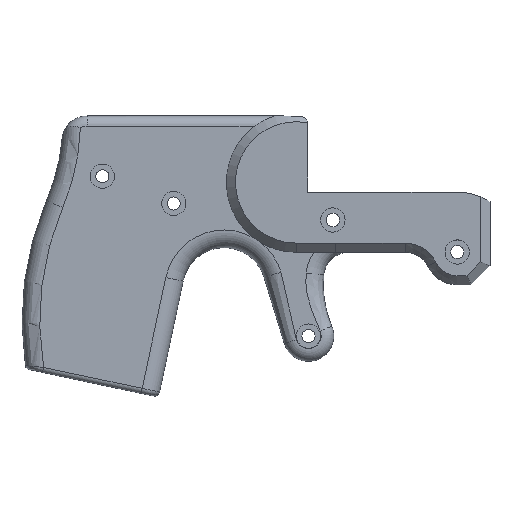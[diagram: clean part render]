
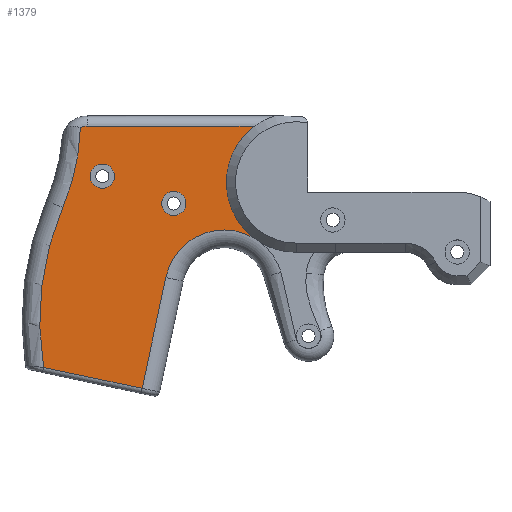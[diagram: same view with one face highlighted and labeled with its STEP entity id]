
A CAD part, top view. The second image highlights one B-rep face of the part: STEP entity #1379.
In plain terms, the highlighted planar face has unit normal (0, 0, 1).
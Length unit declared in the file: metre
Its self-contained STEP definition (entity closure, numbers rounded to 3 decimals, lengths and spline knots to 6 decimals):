
#89=LINE('',#2072,#190);
#90=LINE('',#2074,#191);
#91=LINE('',#2080,#192);
#190=VECTOR('',#1650,1.);
#191=VECTOR('',#1651,1.);
#192=VECTOR('',#1656,1.);
#291=ORIENTED_EDGE('',*,*,#693,.F.);
#292=ORIENTED_EDGE('',*,*,#694,.F.);
#293=ORIENTED_EDGE('',*,*,#695,.T.);
#294=ORIENTED_EDGE('',*,*,#696,.T.);
#295=ORIENTED_EDGE('',*,*,#697,.T.);
#296=ORIENTED_EDGE('',*,*,#698,.T.);
#297=ORIENTED_EDGE('',*,*,#699,.F.);
#298=ORIENTED_EDGE('',*,*,#700,.T.);
#299=ORIENTED_EDGE('',*,*,#701,.T.);
#300=ORIENTED_EDGE('',*,*,#702,.T.);
#693=EDGE_CURVE('',#894,#894,#1030,.T.);
#694=EDGE_CURVE('',#895,#895,#1031,.T.);
#695=EDGE_CURVE('',#896,#897,#1032,.T.);
#696=EDGE_CURVE('',#897,#898,#89,.T.);
#697=EDGE_CURVE('',#898,#899,#90,.T.);
#698=EDGE_CURVE('',#899,#900,#1033,.F.);
#699=EDGE_CURVE('',#901,#900,#1034,.T.);
#700=EDGE_CURVE('',#901,#902,#91,.F.);
#701=EDGE_CURVE('',#902,#903,#1035,.T.);
#702=EDGE_CURVE('',#903,#896,#1036,.F.);
#894=VERTEX_POINT('',#2066);
#895=VERTEX_POINT('',#2068);
#896=VERTEX_POINT('',#2070);
#897=VERTEX_POINT('',#2071);
#898=VERTEX_POINT('',#2073);
#899=VERTEX_POINT('',#2075);
#900=VERTEX_POINT('',#2077);
#901=VERTEX_POINT('',#2079);
#902=VERTEX_POINT('',#2081);
#903=VERTEX_POINT('',#2083);
#1030=CIRCLE('',#1481,0.003048);
#1031=CIRCLE('',#1482,0.003048);
#1032=CIRCLE('',#1483,0.071755);
#1033=CIRCLE('',#1484,0.014949);
#1034=CIRCLE('',#1485,0.017526);
#1035=CIRCLE('',#1486,0.00381);
#1036=CIRCLE('',#1487,0.055245);
#1101=EDGE_LOOP('',(#291));
#1102=EDGE_LOOP('',(#292));
#1103=EDGE_LOOP('',(#293,#294,#295,#296,#297,#298,#299,#300));
#1220=FACE_BOUND('',#1101,.T.);
#1221=FACE_BOUND('',#1102,.T.);
#1222=FACE_BOUND('',#1103,.T.);
#1339=PLANE('',#1480);
#1379=ADVANCED_FACE('',(#1220,#1221,#1222),#1339,.T.);
#1480=AXIS2_PLACEMENT_3D('',#2064,#1642,#1643);
#1481=AXIS2_PLACEMENT_3D('',#2065,#1644,#1645);
#1482=AXIS2_PLACEMENT_3D('',#2067,#1646,#1647);
#1483=AXIS2_PLACEMENT_3D('',#2069,#1648,#1649);
#1484=AXIS2_PLACEMENT_3D('',#2076,#1652,#1653);
#1485=AXIS2_PLACEMENT_3D('',#2078,#1654,#1655);
#1486=AXIS2_PLACEMENT_3D('',#2082,#1657,#1658);
#1487=AXIS2_PLACEMENT_3D('',#2084,#1659,#1660);
#1642=DIRECTION('',(0.,0.,1.));
#1643=DIRECTION('',(1.,0.,0.));
#1644=DIRECTION('',(0.,0.,1.));
#1645=DIRECTION('',(1.,0.,0.));
#1646=DIRECTION('',(0.,0.,1.));
#1647=DIRECTION('',(1.,0.,0.));
#1648=DIRECTION('',(0.,0.,1.));
#1649=DIRECTION('',(1.,0.,0.));
#1650=DIRECTION('',(0.978,-0.208,0.));
#1651=DIRECTION('',(0.208,0.978,0.));
#1652=DIRECTION('',(0.,0.,1.));
#1653=DIRECTION('',(1.,0.,0.));
#1654=DIRECTION('',(0.,0.,1.));
#1655=DIRECTION('',(1.,0.,0.));
#1656=DIRECTION('',(1.,0.,0.));
#1657=DIRECTION('',(0.,0.,1.));
#1658=DIRECTION('',(1.,0.,0.));
#1659=DIRECTION('',(0.,0.,1.));
#1660=DIRECTION('',(1.,0.,0.));
#2064=CARTESIAN_POINT('',(-0.008016,0.021885,0.005));
#2065=CARTESIAN_POINT('',(-0.050147,0.03645,0.005));
#2066=CARTESIAN_POINT('',(-0.047099,0.03645,0.005));
#2067=CARTESIAN_POINT('',(-0.032246,0.02961,0.005));
#2068=CARTESIAN_POINT('',(-0.029198,0.02961,0.005));
#2069=CARTESIAN_POINT('',(0.005865,0.00034,0.005));
#2070=CARTESIAN_POINT('',(-0.060099,0.028581,0.005));
#2071=CARTESIAN_POINT('',(-0.064897,-0.011553,0.005));
#2072=CARTESIAN_POINT('',(-0.040165,-0.01681,0.005));
#2073=CARTESIAN_POINT('',(-0.040165,-0.01681,0.005));
#2074=CARTESIAN_POINT('',(-0.034241,0.01106,0.005));
#2075=CARTESIAN_POINT('',(-0.034246,0.011035,0.005));
#2076=CARTESIAN_POINT('',(-0.019608,0.008005,0.005));
#2077=CARTESIAN_POINT('',(-0.01206,0.020909,0.005));
#2078=CARTESIAN_POINT('',(-0.001494,0.034891,0.005));
#2079=CARTESIAN_POINT('',(-0.011818,0.049054,0.005));
#2080=CARTESIAN_POINT('',(-0.053961,0.049054,0.005));
#2081=CARTESIAN_POINT('',(-0.053961,0.049054,0.005));
#2082=CARTESIAN_POINT('',(-0.053961,0.045244,0.005));
#2083=CARTESIAN_POINT('',(-0.055665,0.048651,0.005));
#2084=CARTESIAN_POINT('',(-0.110885,0.050324,0.005));
